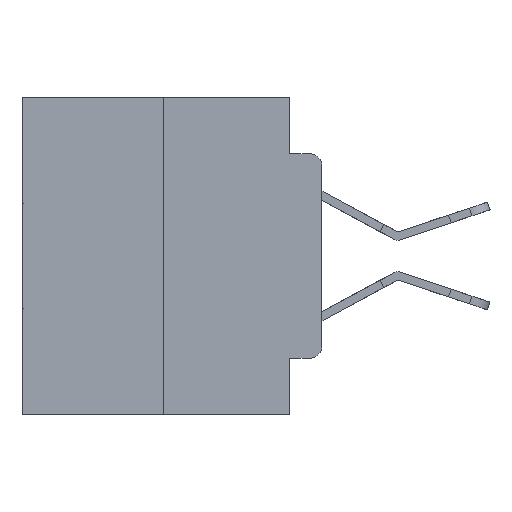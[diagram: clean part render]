
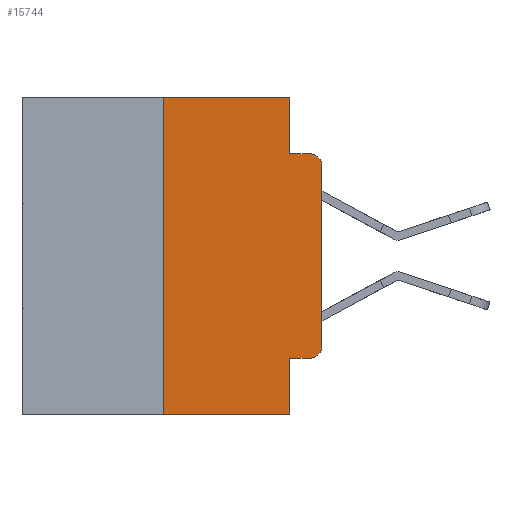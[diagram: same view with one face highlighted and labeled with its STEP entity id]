
A CAD part, left-side view. The second image highlights one B-rep face of the part: STEP entity #15744.
In plain terms, the highlighted planar face has unit normal (-1, 0, 0).
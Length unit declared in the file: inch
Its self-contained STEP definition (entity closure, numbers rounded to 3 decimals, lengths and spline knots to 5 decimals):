
#446 = CARTESIAN_POINT ( 'NONE',  ( 0., 0.051, -0.4115 ) ) ;
#493 = CARTESIAN_POINT ( 'NONE',  ( 0., 0.02, -0.0885 ) ) ;
#1009 = ORIENTED_EDGE ( 'NONE', *, *, #8501, .T. ) ;
#1774 = EDGE_CURVE ( 'NONE', #10444, #2631, #24751, .T. ) ;
#2003 = VERTEX_POINT ( 'NONE', #17295 ) ;
#2259 = AXIS2_PLACEMENT_3D ( 'NONE', #25501, #25405, #26889 ) ;
#2552 = ORIENTED_EDGE ( 'NONE', *, *, #20120, .F. ) ;
#2631 = VERTEX_POINT ( 'NONE', #493 ) ;
#2870 = DIRECTION ( 'NONE',  ( 0., -1., 0. ) ) ;
#4041 = ORIENTED_EDGE ( 'NONE', *, *, #15814, .F. ) ;
#4280 = VECTOR ( 'NONE', #19499, 39.37008 ) ;
#4881 = CARTESIAN_POINT ( 'NONE',  ( 0., 0.25, 0. ) ) ;
#6743 = LINE ( 'NONE', #10669, #18691 ) ;
#7146 = EDGE_CURVE ( 'NONE', #17874, #18746, #26970, .T. ) ;
#7447 = DIRECTION ( 'NONE',  ( -1., 0., 0. ) ) ;
#7767 = LINE ( 'NONE', #15311, #24452 ) ;
#7805 = ORIENTED_EDGE ( 'NONE', *, *, #24568, .T. ) ;
#8079 = CARTESIAN_POINT ( 'NONE',  ( 0., 0.473, 0. ) ) ;
#8199 = VERTEX_POINT ( 'NONE', #28628 ) ;
#8501 = EDGE_CURVE ( 'NONE', #24755, #10444, #23273, .T. ) ;
#8673 = LINE ( 'NONE', #446, #26794 ) ;
#9240 = EDGE_LOOP ( 'NONE', ( #1009, #14441, #22985, #18193, #10755, #2552, #27753, #4041, #7805, #27393 ) ) ;
#9613 = AXIS2_PLACEMENT_3D ( 'NONE', #8079, #12852, #29340 ) ;
#10275 = EDGE_CURVE ( 'NONE', #2003, #24755, #30086, .T. ) ;
#10444 = VERTEX_POINT ( 'NONE', #26891 ) ;
#10469 = PLANE ( 'NONE',  #9613 ) ;
#10641 = VECTOR ( 'NONE', #23924, 39.37008 ) ;
#10669 = CARTESIAN_POINT ( 'NONE',  ( 0., 0.051, 0. ) ) ;
#10755 = ORIENTED_EDGE ( 'NONE', *, *, #28800, .F. ) ;
#11432 = CARTESIAN_POINT ( 'NONE',  ( 0., 0.051, -0.0885 ) ) ;
#12010 = VERTEX_POINT ( 'NONE', #26500 ) ;
#12127 = CARTESIAN_POINT ( 'NONE',  ( 0., 0.25, -0.5 ) ) ;
#12852 = DIRECTION ( 'NONE',  ( 1., 0., 0. ) ) ;
#12857 = LINE ( 'NONE', #14238, #30171 ) ;
#13691 = CARTESIAN_POINT ( 'NONE',  ( 0., 0.051, 0. ) ) ;
#14238 = CARTESIAN_POINT ( 'NONE',  ( 0., 0.473, -0.5 ) ) ;
#14441 = ORIENTED_EDGE ( 'NONE', *, *, #1774, .T. ) ;
#14719 = CARTESIAN_POINT ( 'NONE',  ( 0., 0., 0. ) ) ;
#15311 = CARTESIAN_POINT ( 'NONE',  ( 0., 0.473, 0. ) ) ;
#15473 = DIRECTION ( 'NONE',  ( 0., 0., -1. ) ) ;
#15744 = ADVANCED_FACE ( 'NONE', ( #27125 ), #10469, .F. ) ;
#15814 = EDGE_CURVE ( 'NONE', #22566, #8199, #6743, .T. ) ;
#16237 = LINE ( 'NONE', #4881, #10641 ) ;
#16674 = VECTOR ( 'NONE', #27909, 39.37008 ) ;
#17093 = AXIS2_PLACEMENT_3D ( 'NONE', #21692, #7447, #24035 ) ;
#17295 = CARTESIAN_POINT ( 'NONE',  ( 0., 0.02, -0.4115 ) ) ;
#17688 = DIRECTION ( 'NONE',  ( 0., -1., 0. ) ) ;
#17874 = VERTEX_POINT ( 'NONE', #13691 ) ;
#17914 = EDGE_CURVE ( 'NONE', #18746, #2631, #27712, .T. ) ;
#17919 = CARTESIAN_POINT ( 'NONE',  ( 0., 0.051, 0. ) ) ;
#18193 = ORIENTED_EDGE ( 'NONE', *, *, #7146, .F. ) ;
#18691 = VECTOR ( 'NONE', #15473, 39.37008 ) ;
#18746 = VERTEX_POINT ( 'NONE', #18978 ) ;
#18978 = CARTESIAN_POINT ( 'NONE',  ( 0., 0.051, -0.0885 ) ) ;
#19038 = DIRECTION ( 'NONE',  ( 0., -1., 0. ) ) ;
#19499 = DIRECTION ( 'NONE',  ( 0., 0., 1. ) ) ;
#20120 = EDGE_CURVE ( 'NONE', #22326, #12010, #16237, .T. ) ;
#20460 = CARTESIAN_POINT ( 'NONE',  ( 0., 0.051, -0.4115 ) ) ;
#20760 = VECTOR ( 'NONE', #22672, 39.37008 ) ;
#21692 = CARTESIAN_POINT ( 'NONE',  ( 0., 0.02, -0.3915 ) ) ;
#22171 = EDGE_CURVE ( 'NONE', #22326, #8199, #12857, .T. ) ;
#22326 = VERTEX_POINT ( 'NONE', #12127 ) ;
#22566 = VERTEX_POINT ( 'NONE', #20460 ) ;
#22672 = DIRECTION ( 'NONE',  ( 0., 0., -1. ) ) ;
#22985 = ORIENTED_EDGE ( 'NONE', *, *, #17914, .F. ) ;
#23273 = LINE ( 'NONE', #14719, #4280 ) ;
#23924 = DIRECTION ( 'NONE',  ( 0., 0., 1. ) ) ;
#24035 = DIRECTION ( 'NONE',  ( 0., 0., -1. ) ) ;
#24452 = VECTOR ( 'NONE', #17688, 39.37008 ) ;
#24568 = EDGE_CURVE ( 'NONE', #22566, #2003, #8673, .T. ) ;
#24751 = CIRCLE ( 'NONE', #2259, 0.02 ) ;
#24755 = VERTEX_POINT ( 'NONE', #24877 ) ;
#24877 = CARTESIAN_POINT ( 'NONE',  ( 0., 0., -0.3915 ) ) ;
#25405 = DIRECTION ( 'NONE',  ( -1., 0., 0. ) ) ;
#25501 = CARTESIAN_POINT ( 'NONE',  ( 0., 0.02, -0.1085 ) ) ;
#26500 = CARTESIAN_POINT ( 'NONE',  ( 0., 0.25, 0. ) ) ;
#26794 = VECTOR ( 'NONE', #2870, 39.37008 ) ;
#26889 = DIRECTION ( 'NONE',  ( 0., 0., -1. ) ) ;
#26891 = CARTESIAN_POINT ( 'NONE',  ( 0., 0., -0.1085 ) ) ;
#26970 = LINE ( 'NONE', #17919, #20760 ) ;
#27125 = FACE_OUTER_BOUND ( 'NONE', #9240, .T. ) ;
#27393 = ORIENTED_EDGE ( 'NONE', *, *, #10275, .T. ) ;
#27712 = LINE ( 'NONE', #11432, #16674 ) ;
#27753 = ORIENTED_EDGE ( 'NONE', *, *, #22171, .T. ) ;
#27909 = DIRECTION ( 'NONE',  ( 0., -1., 0. ) ) ;
#28628 = CARTESIAN_POINT ( 'NONE',  ( 0., 0.051, -0.5 ) ) ;
#28800 = EDGE_CURVE ( 'NONE', #12010, #17874, #7767, .T. ) ;
#29340 = DIRECTION ( 'NONE',  ( 0., 0., -1. ) ) ;
#30086 = CIRCLE ( 'NONE', #17093, 0.02 ) ;
#30171 = VECTOR ( 'NONE', #19038, 39.37008 ) ;
